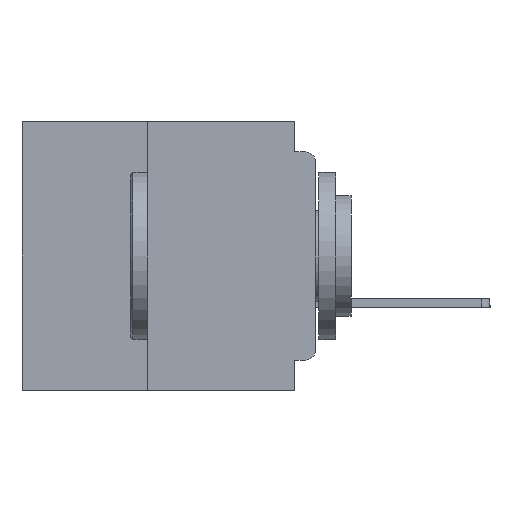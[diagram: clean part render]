
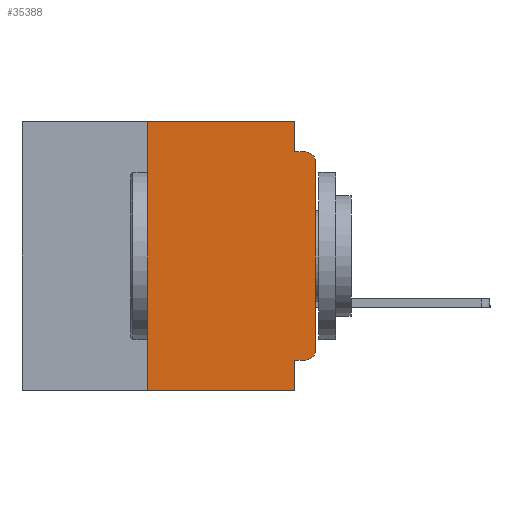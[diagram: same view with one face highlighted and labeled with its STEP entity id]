
A CAD part, left-side view. The second image highlights one B-rep face of the part: STEP entity #35388.
In plain terms, the highlighted planar face has unit normal (-1, 0, 0).
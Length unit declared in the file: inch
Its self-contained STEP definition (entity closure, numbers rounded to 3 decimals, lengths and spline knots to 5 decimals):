
#525 = EDGE_CURVE ( 'NONE', #41330, #2163, #31330, .T. ) ;
#535 = DIRECTION ( 'NONE',  ( 0., -1., 0. ) ) ;
#819 = EDGE_CURVE ( 'NONE', #930, #38053, #4292, .T. ) ;
#848 = ORIENTED_EDGE ( 'NONE', *, *, #52828, .F. ) ;
#930 = VERTEX_POINT ( 'NONE', #56593 ) ;
#1101 = DIRECTION ( 'NONE',  ( -1., 0., 0. ) ) ;
#1109 = EDGE_CURVE ( 'NONE', #57413, #45392, #56356, .T. ) ;
#2163 = VERTEX_POINT ( 'NONE', #24115 ) ;
#2544 = VECTOR ( 'NONE', #45871, 39.37008 ) ;
#4292 = LINE ( 'NONE', #23076, #49278 ) ;
#5438 = VECTOR ( 'NONE', #47876, 39.37008 ) ;
#5575 = CARTESIAN_POINT ( 'NONE',  ( 0., 0.031, 0. ) ) ;
#5975 = CARTESIAN_POINT ( 'NONE',  ( 0., 0.437, 0. ) ) ;
#6212 = VECTOR ( 'NONE', #535, 39.37008 ) ;
#6989 = ORIENTED_EDGE ( 'NONE', *, *, #43851, .F. ) ;
#9540 = VECTOR ( 'NONE', #17431, 39.37008 ) ;
#11873 = EDGE_CURVE ( 'NONE', #2163, #44741, #46735, .T. ) ;
#12929 = ORIENTED_EDGE ( 'NONE', *, *, #819, .F. ) ;
#14114 = EDGE_CURVE ( 'NONE', #45645, #930, #15775, .T. ) ;
#14970 = CARTESIAN_POINT ( 'NONE',  ( 0., 0.031, 0. ) ) ;
#15396 = PLANE ( 'NONE',  #48928 ) ;
#15584 = EDGE_CURVE ( 'NONE', #44741, #38053, #30969, .T. ) ;
#15665 = DIRECTION ( 'NONE',  ( 0., 0., 1. ) ) ;
#15775 = LINE ( 'NONE', #5575, #17266 ) ;
#16109 = CARTESIAN_POINT ( 'NONE',  ( 0., 0.015, -0.34 ) ) ;
#17023 = CARTESIAN_POINT ( 'NONE',  ( 0., 0.25, -0.4 ) ) ;
#17266 = VECTOR ( 'NONE', #33532, 39.37008 ) ;
#17431 = DIRECTION ( 'NONE',  ( 0., -1., 0. ) ) ;
#17708 = CARTESIAN_POINT ( 'NONE',  ( 0., 0.25, 0. ) ) ;
#18675 = LINE ( 'NONE', #46861, #6212 ) ;
#18697 = ORIENTED_EDGE ( 'NONE', *, *, #15584, .T. ) ;
#20187 = CARTESIAN_POINT ( 'NONE',  ( 0., 0.25, -0.4 ) ) ;
#20620 = AXIS2_PLACEMENT_3D ( 'NONE', #29086, #1101, #33773 ) ;
#21896 = CARTESIAN_POINT ( 'NONE',  ( 0., 0.437, 0. ) ) ;
#21987 = LINE ( 'NONE', #21896, #9540 ) ;
#22403 = DIRECTION ( 'NONE',  ( 0., -1., 0. ) ) ;
#22823 = CARTESIAN_POINT ( 'NONE',  ( 0., 0., -0.355 ) ) ;
#23076 = CARTESIAN_POINT ( 'NONE',  ( 0., 0., -0.045 ) ) ;
#23947 = AXIS2_PLACEMENT_3D ( 'NONE', #16109, #45624, #39403 ) ;
#24115 = CARTESIAN_POINT ( 'NONE',  ( 0., 0., -0.34 ) ) ;
#24776 = DIRECTION ( 'NONE',  ( 1., 0., 0. ) ) ;
#25237 = CARTESIAN_POINT ( 'NONE',  ( 0., 0., 0. ) ) ;
#25284 = FACE_OUTER_BOUND ( 'NONE', #46422, .T. ) ;
#27176 = VERTEX_POINT ( 'NONE', #17708 ) ;
#29086 = CARTESIAN_POINT ( 'NONE',  ( 0., 0.015, -0.06 ) ) ;
#30969 = CIRCLE ( 'NONE', #20620, 0.015 ) ;
#31068 = CARTESIAN_POINT ( 'NONE',  ( 0., 0., -0.06 ) ) ;
#31330 = CIRCLE ( 'NONE', #23947, 0.015 ) ;
#31507 = DIRECTION ( 'NONE',  ( 0., 0., -1. ) ) ;
#31870 = CARTESIAN_POINT ( 'NONE',  ( 0., 0.031, -0.4 ) ) ;
#33532 = DIRECTION ( 'NONE',  ( 0., 0., -1. ) ) ;
#33773 = DIRECTION ( 'NONE',  ( 0., 0., -1. ) ) ;
#35388 = ADVANCED_FACE ( 'NONE', ( #25284 ), #15396, .F. ) ;
#38053 = VERTEX_POINT ( 'NONE', #45418 ) ;
#38243 = ORIENTED_EDGE ( 'NONE', *, *, #14114, .F. ) ;
#39403 = DIRECTION ( 'NONE',  ( 0., 0., -1. ) ) ;
#39737 = LINE ( 'NONE', #22823, #2544 ) ;
#41330 = VERTEX_POINT ( 'NONE', #52609 ) ;
#41646 = ORIENTED_EDGE ( 'NONE', *, *, #54300, .T. ) ;
#42825 = ORIENTED_EDGE ( 'NONE', *, *, #11873, .T. ) ;
#43851 = EDGE_CURVE ( 'NONE', #45798, #27176, #54662, .T. ) ;
#44251 = VECTOR ( 'NONE', #31507, 39.37008 ) ;
#44741 = VERTEX_POINT ( 'NONE', #31068 ) ;
#45300 = VECTOR ( 'NONE', #15665, 39.37008 ) ;
#45392 = VERTEX_POINT ( 'NONE', #50293 ) ;
#45418 = CARTESIAN_POINT ( 'NONE',  ( 0., 0.015, -0.045 ) ) ;
#45624 = DIRECTION ( 'NONE',  ( -1., 0., 0. ) ) ;
#45645 = VERTEX_POINT ( 'NONE', #14970 ) ;
#45798 = VERTEX_POINT ( 'NONE', #17023 ) ;
#45850 = EDGE_CURVE ( 'NONE', #27176, #45645, #21987, .T. ) ;
#45871 = DIRECTION ( 'NONE',  ( 0., 1., 0. ) ) ;
#46422 = EDGE_LOOP ( 'NONE', ( #42825, #18697, #12929, #38243, #55452, #6989, #41646, #58566, #848, #54415 ) ) ;
#46735 = LINE ( 'NONE', #25237, #45300 ) ;
#46861 = CARTESIAN_POINT ( 'NONE',  ( 0., 0.437, -0.4 ) ) ;
#47691 = CARTESIAN_POINT ( 'NONE',  ( 0., 0.031, -0.355 ) ) ;
#47876 = DIRECTION ( 'NONE',  ( 0., 0., 1. ) ) ;
#48928 = AXIS2_PLACEMENT_3D ( 'NONE', #5975, #24776, #56916 ) ;
#49278 = VECTOR ( 'NONE', #22403, 39.37008 ) ;
#50293 = CARTESIAN_POINT ( 'NONE',  ( 0., 0.031, -0.4 ) ) ;
#52609 = CARTESIAN_POINT ( 'NONE',  ( 0., 0.015, -0.355 ) ) ;
#52828 = EDGE_CURVE ( 'NONE', #41330, #57413, #39737, .T. ) ;
#54300 = EDGE_CURVE ( 'NONE', #45798, #45392, #18675, .T. ) ;
#54415 = ORIENTED_EDGE ( 'NONE', *, *, #525, .T. ) ;
#54662 = LINE ( 'NONE', #20187, #5438 ) ;
#55452 = ORIENTED_EDGE ( 'NONE', *, *, #45850, .F. ) ;
#56356 = LINE ( 'NONE', #31870, #44251 ) ;
#56593 = CARTESIAN_POINT ( 'NONE',  ( 0., 0.031, -0.045 ) ) ;
#56916 = DIRECTION ( 'NONE',  ( 0., 0., -1. ) ) ;
#57413 = VERTEX_POINT ( 'NONE', #47691 ) ;
#58566 = ORIENTED_EDGE ( 'NONE', *, *, #1109, .F. ) ;
